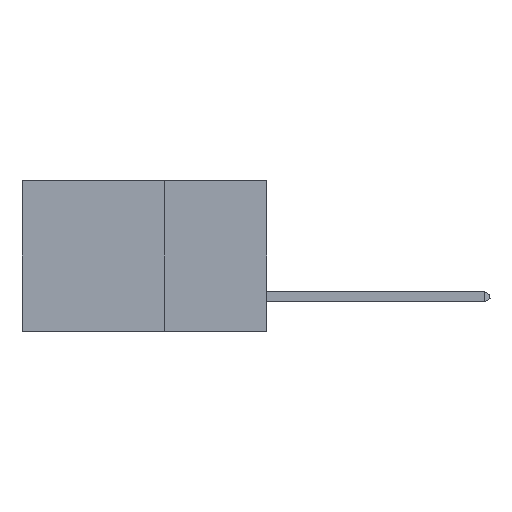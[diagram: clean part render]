
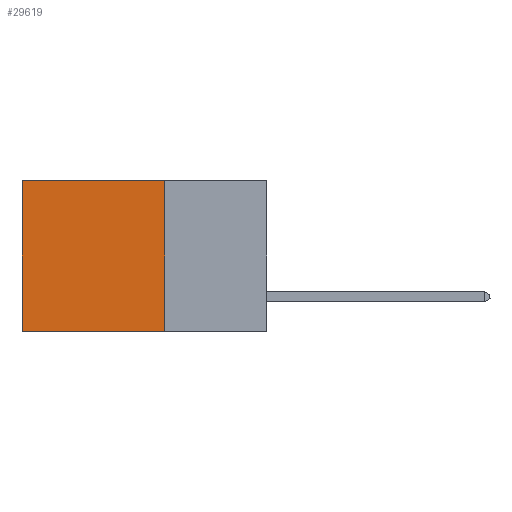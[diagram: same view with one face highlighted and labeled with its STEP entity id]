
A CAD part, left-side view. The second image highlights one B-rep face of the part: STEP entity #29619.
In plain terms, the highlighted planar face has unit normal (-1, 0, 0).
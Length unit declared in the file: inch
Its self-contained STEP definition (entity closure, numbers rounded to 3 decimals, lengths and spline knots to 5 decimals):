
#1336 = CARTESIAN_POINT ( 'NONE',  ( 0.2875, 0.6, -0.37 ) ) ;
#1492 = EDGE_CURVE ( 'NONE', #38185, #16438, #32915, .T. ) ;
#4278 = CARTESIAN_POINT ( 'NONE',  ( 0.2875, 0.25, 0. ) ) ;
#5460 = EDGE_CURVE ( 'NONE', #38185, #41138, #21010, .T. ) ;
#8252 = DIRECTION ( 'NONE',  ( 0., 0., -1. ) ) ;
#8498 = DIRECTION ( 'NONE',  ( 0., 1., 0. ) ) ;
#11174 = CARTESIAN_POINT ( 'NONE',  ( 0.2875, 0.6, 0. ) ) ;
#12267 = PLANE ( 'NONE',  #33806 ) ;
#13155 = LINE ( 'NONE', #19229, #21047 ) ;
#16438 = VERTEX_POINT ( 'NONE', #46982 ) ;
#18500 = FACE_OUTER_BOUND ( 'NONE', #46458, .T. ) ;
#19161 = ORIENTED_EDGE ( 'NONE', *, *, #5460, .T. ) ;
#19229 = CARTESIAN_POINT ( 'NONE',  ( 0.2875, 0.25, -0.37 ) ) ;
#21010 = LINE ( 'NONE', #46338, #36802 ) ;
#21047 = VECTOR ( 'NONE', #8498, 39.37008 ) ;
#27148 = EDGE_CURVE ( 'NONE', #41138, #36217, #40912, .T. ) ;
#27812 = DIRECTION ( 'NONE',  ( 1., 0., 0. ) ) ;
#27817 = EDGE_CURVE ( 'NONE', #16438, #36217, #13155, .T. ) ;
#29261 = ORIENTED_EDGE ( 'NONE', *, *, #27817, .F. ) ;
#29491 = CARTESIAN_POINT ( 'NONE',  ( 0.2875, 0.25, 0. ) ) ;
#29619 = ADVANCED_FACE ( 'NONE', ( #18500 ), #12267, .F. ) ;
#32061 = CARTESIAN_POINT ( 'NONE',  ( 0.2875, 0.25, 0. ) ) ;
#32848 = ORIENTED_EDGE ( 'NONE', *, *, #27148, .T. ) ;
#32915 = LINE ( 'NONE', #4278, #47413 ) ;
#33806 = AXIS2_PLACEMENT_3D ( 'NONE', #29491, #27812, #48766 ) ;
#36217 = VERTEX_POINT ( 'NONE', #1336 ) ;
#36802 = VECTOR ( 'NONE', #42817, 39.37008 ) ;
#38185 = VERTEX_POINT ( 'NONE', #32061 ) ;
#38516 = DIRECTION ( 'NONE',  ( 0., 0., -1. ) ) ;
#40651 = ORIENTED_EDGE ( 'NONE', *, *, #1492, .F. ) ;
#40912 = LINE ( 'NONE', #42222, #46325 ) ;
#41138 = VERTEX_POINT ( 'NONE', #11174 ) ;
#42222 = CARTESIAN_POINT ( 'NONE',  ( 0.2875, 0.6, 0. ) ) ;
#42817 = DIRECTION ( 'NONE',  ( 0., 1., 0. ) ) ;
#46325 = VECTOR ( 'NONE', #38516, 39.37008 ) ;
#46338 = CARTESIAN_POINT ( 'NONE',  ( 0.2875, 0.25, 0. ) ) ;
#46458 = EDGE_LOOP ( 'NONE', ( #32848, #29261, #40651, #19161 ) ) ;
#46982 = CARTESIAN_POINT ( 'NONE',  ( 0.2875, 0.25, -0.37 ) ) ;
#47413 = VECTOR ( 'NONE', #8252, 39.37008 ) ;
#48766 = DIRECTION ( 'NONE',  ( 0., 0., -1. ) ) ;
